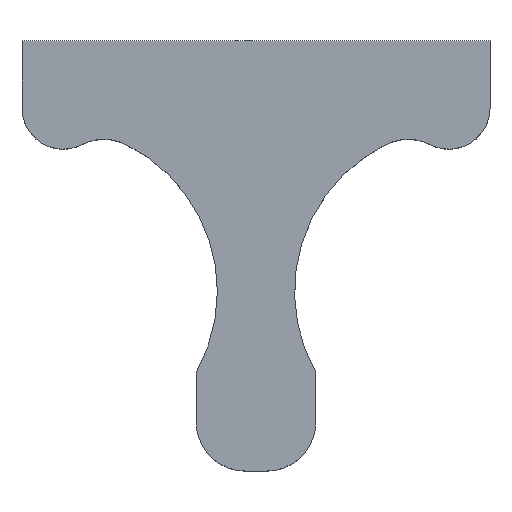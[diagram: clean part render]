
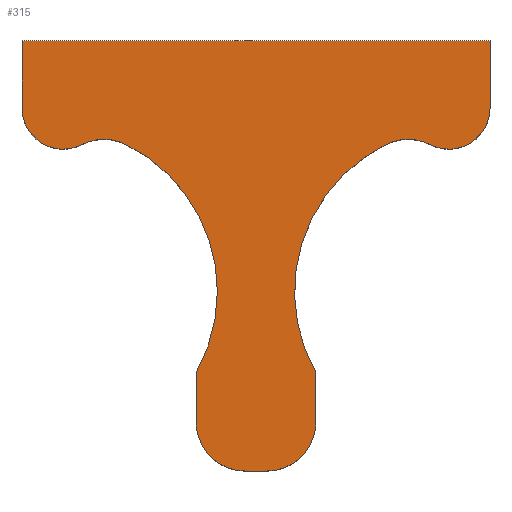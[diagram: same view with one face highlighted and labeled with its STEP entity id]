
A CAD part, top view. The second image highlights one B-rep face of the part: STEP entity #315.
In plain terms, the highlighted planar face has unit normal (0, 0, 1).
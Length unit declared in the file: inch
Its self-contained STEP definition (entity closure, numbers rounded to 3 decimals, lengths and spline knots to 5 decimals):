
#12 = EDGE_CURVE ( 'NONE', #204, #363, #301, .T. ) ;
#14 = DIRECTION ( 'NONE',  ( 0., 0., 1. ) ) ;
#17 = AXIS2_PLACEMENT_3D ( 'NONE', #470, #14, #563 ) ;
#20 = VERTEX_POINT ( 'NONE', #534 ) ;
#24 = EDGE_CURVE ( 'NONE', #46, #204, #52, .T. ) ;
#29 = CIRCLE ( 'NONE', #97, 0.03 ) ;
#37 = CARTESIAN_POINT ( 'NONE',  ( -0.1235, -0.15277, 0.026 ) ) ;
#38 = LINE ( 'NONE', #488, #371 ) ;
#46 = VERTEX_POINT ( 'NONE', #209 ) ;
#47 = DIRECTION ( 'NONE',  ( 0., 1., 0. ) ) ;
#49 = CARTESIAN_POINT ( 'NONE',  ( -0.1175, -0.041, 0.026 ) ) ;
#52 = CIRCLE ( 'NONE', #155, 0.03 ) ;
#54 = ORIENTED_EDGE ( 'NONE', *, *, #345, .T. ) ;
#62 = VERTEX_POINT ( 'NONE', #578 ) ;
#63 = EDGE_CURVE ( 'NONE', #366, #337, #443, .T. ) ;
#69 = VECTOR ( 'NONE', #482, 39.37008 ) ;
#70 = DIRECTION ( 'NONE',  ( 0., 0., 1. ) ) ;
#83 = DIRECTION ( 'NONE',  ( -1., 0., 0. ) ) ;
#84 = CARTESIAN_POINT ( 'NONE',  ( -0.1425, 0., 0.026 ) ) ;
#85 = VERTEX_POINT ( 'NONE', #167 ) ;
#91 = LINE ( 'NONE', #467, #316 ) ;
#93 = CIRCLE ( 'NONE', #390, 0.025 ) ;
#95 = CARTESIAN_POINT ( 'NONE',  ( 0.09252, -0.09, 0.026 ) ) ;
#97 = AXIS2_PLACEMENT_3D ( 'NONE', #405, #587, #306 ) ;
#99 = DIRECTION ( 'NONE',  ( 1., 0., 0. ) ) ;
#104 = VERTEX_POINT ( 'NONE', #84 ) ;
#114 = CARTESIAN_POINT ( 'NONE',  ( -0.0065, -0.262, 0.026 ) ) ;
#120 = CARTESIAN_POINT ( 'NONE',  ( -0.1175, -0.041, 0.026 ) ) ;
#126 = EDGE_CURVE ( 'NONE', #85, #62, #29, .T. ) ;
#130 = CARTESIAN_POINT ( 'NONE',  ( 0.0065, -0.262, 0.026 ) ) ;
#134 = EDGE_CURVE ( 'NONE', #62, #372, #589, .T. ) ;
#135 = VERTEX_POINT ( 'NONE', #496 ) ;
#136 = DIRECTION ( 'NONE',  ( 0., 0., 1. ) ) ;
#137 = DIRECTION ( 'NONE',  ( 0., 0., -1. ) ) ;
#138 = DIRECTION ( 'NONE',  ( 0., 0., 1. ) ) ;
#142 = CARTESIAN_POINT ( 'NONE',  ( 0.0365, -0.20208, 0.026 ) ) ;
#143 = AXIS2_PLACEMENT_3D ( 'NONE', #37, #446, #83 ) ;
#145 = AXIS2_PLACEMENT_3D ( 'NONE', #495, #299, #537 ) ;
#154 = DIRECTION ( 'NONE',  ( 0., -1., 0. ) ) ;
#155 = AXIS2_PLACEMENT_3D ( 'NONE', #309, #70, #402 ) ;
#165 = CARTESIAN_POINT ( 'NONE',  ( 0.1425, 0., 0.026 ) ) ;
#167 = CARTESIAN_POINT ( 'NONE',  ( -0.10615, -0.06327, 0.026 ) ) ;
#171 = VERTEX_POINT ( 'NONE', #413 ) ;
#201 = VECTOR ( 'NONE', #154, 39.37008 ) ;
#204 = VERTEX_POINT ( 'NONE', #403 ) ;
#208 = EDGE_CURVE ( 'NONE', #291, #135, #259, .T. ) ;
#209 = CARTESIAN_POINT ( 'NONE',  ( -0.0365, -0.232, 0.026 ) ) ;
#217 = CIRCLE ( 'NONE', #553, 0.025 ) ;
#225 = EDGE_CURVE ( 'NONE', #20, #366, #429, .T. ) ;
#232 = ORIENTED_EDGE ( 'NONE', *, *, #12, .T. ) ;
#240 = FACE_OUTER_BOUND ( 'NONE', #475, .T. ) ;
#244 = ORIENTED_EDGE ( 'NONE', *, *, #379, .T. ) ;
#259 = LINE ( 'NONE', #165, #562 ) ;
#261 = AXIS2_PLACEMENT_3D ( 'NONE', #49, #136, #281 ) ;
#268 = CARTESIAN_POINT ( 'NONE',  ( 0.1425, -0.041, 0.026 ) ) ;
#270 = PLANE ( 'NONE',  #261 ) ;
#272 = ORIENTED_EDGE ( 'NONE', *, *, #24, .T. ) ;
#275 = AXIS2_PLACEMENT_3D ( 'NONE', #95, #519, #99 ) ;
#276 = ORIENTED_EDGE ( 'NONE', *, *, #577, .T. ) ;
#281 = DIRECTION ( 'NONE',  ( 1., 0., 0. ) ) ;
#289 = LINE ( 'NONE', #440, #201 ) ;
#291 = VERTEX_POINT ( 'NONE', #268 ) ;
#293 = ORIENTED_EDGE ( 'NONE', *, *, #208, .T. ) ;
#299 = DIRECTION ( 'NONE',  ( 0., 0., -1. ) ) ;
#301 = LINE ( 'NONE', #114, #69 ) ;
#306 = DIRECTION ( 'NONE',  ( -1., 0., 0. ) ) ;
#309 = CARTESIAN_POINT ( 'NONE',  ( -0.0065, -0.232, 0.026 ) ) ;
#315 = ADVANCED_FACE ( 'NONE', ( #240 ), #270, .T. ) ;
#316 = VECTOR ( 'NONE', #421, 39.37008 ) ;
#317 = CARTESIAN_POINT ( 'NONE',  ( -0.0235, -0.15277, 0.026 ) ) ;
#318 = ORIENTED_EDGE ( 'NONE', *, *, #570, .T. ) ;
#323 = DIRECTION ( 'NONE',  ( -1., 0., 0. ) ) ;
#326 = CIRCLE ( 'NONE', #275, 0.03 ) ;
#328 = CARTESIAN_POINT ( 'NONE',  ( 0.1175, -0.041, 0.026 ) ) ;
#331 = ORIENTED_EDGE ( 'NONE', *, *, #490, .T. ) ;
#336 = AXIS2_PLACEMENT_3D ( 'NONE', #484, #137, #422 ) ;
#337 = VERTEX_POINT ( 'NONE', #511 ) ;
#345 = EDGE_CURVE ( 'NONE', #510, #46, #91, .T. ) ;
#347 = CIRCLE ( 'NONE', #17, 0.03 ) ;
#355 = DIRECTION ( 'NONE',  ( 0., 0., 1. ) ) ;
#363 = VERTEX_POINT ( 'NONE', #130 ) ;
#366 = VERTEX_POINT ( 'NONE', #142 ) ;
#369 = ORIENTED_EDGE ( 'NONE', *, *, #134, .T. ) ;
#371 = VECTOR ( 'NONE', #492, 39.37008 ) ;
#372 = VERTEX_POINT ( 'NONE', #317 ) ;
#379 = EDGE_CURVE ( 'NONE', #171, #291, #93, .T. ) ;
#380 = ORIENTED_EDGE ( 'NONE', *, *, #387, .T. ) ;
#387 = EDGE_CURVE ( 'NONE', #337, #171, #326, .T. ) ;
#390 = AXIS2_PLACEMENT_3D ( 'NONE', #328, #138, #323 ) ;
#402 = DIRECTION ( 'NONE',  ( 1., 0., 0. ) ) ;
#403 = CARTESIAN_POINT ( 'NONE',  ( -0.0065, -0.262, 0.026 ) ) ;
#405 = CARTESIAN_POINT ( 'NONE',  ( -0.09252, -0.09, 0.026 ) ) ;
#413 = CARTESIAN_POINT ( 'NONE',  ( 0.10615, -0.06327, 0.026 ) ) ;
#421 = DIRECTION ( 'NONE',  ( 0., -1., 0. ) ) ;
#422 = DIRECTION ( 'NONE',  ( -1., 0., 0. ) ) ;
#429 = LINE ( 'NONE', #515, #501 ) ;
#432 = EDGE_CURVE ( 'NONE', #104, #568, #289, .T. ) ;
#440 = CARTESIAN_POINT ( 'NONE',  ( -0.1425, 0., 0.026 ) ) ;
#443 = CIRCLE ( 'NONE', #145, 0.1 ) ;
#446 = DIRECTION ( 'NONE',  ( 0., 0., -1. ) ) ;
#447 = DIRECTION ( 'NONE',  ( 1., 0., 0. ) ) ;
#453 = CARTESIAN_POINT ( 'NONE',  ( -0.1425, -0.041, 0.026 ) ) ;
#467 = CARTESIAN_POINT ( 'NONE',  ( -0.0365, -0.20208, 0.026 ) ) ;
#470 = CARTESIAN_POINT ( 'NONE',  ( 0.0065, -0.232, 0.026 ) ) ;
#475 = EDGE_LOOP ( 'NONE', ( #514, #276, #499, #369, #331, #54, #272, #232, #504, #558, #486, #380, #244, #293, #318 ) ) ;
#482 = DIRECTION ( 'NONE',  ( 1., 0., 0. ) ) ;
#484 = CARTESIAN_POINT ( 'NONE',  ( -0.1235, -0.15277, 0.026 ) ) ;
#486 = ORIENTED_EDGE ( 'NONE', *, *, #63, .T. ) ;
#488 = CARTESIAN_POINT ( 'NONE',  ( -0.1425, 0., 0.026 ) ) ;
#490 = EDGE_CURVE ( 'NONE', #372, #510, #505, .T. ) ;
#492 = DIRECTION ( 'NONE',  ( -1., 0., 0. ) ) ;
#495 = CARTESIAN_POINT ( 'NONE',  ( 0.1235, -0.15277, 0.026 ) ) ;
#496 = CARTESIAN_POINT ( 'NONE',  ( 0.1425, 0., 0.026 ) ) ;
#499 = ORIENTED_EDGE ( 'NONE', *, *, #126, .T. ) ;
#501 = VECTOR ( 'NONE', #47, 39.37008 ) ;
#504 = ORIENTED_EDGE ( 'NONE', *, *, #533, .T. ) ;
#505 = CIRCLE ( 'NONE', #336, 0.1 ) ;
#510 = VERTEX_POINT ( 'NONE', #517 ) ;
#511 = CARTESIAN_POINT ( 'NONE',  ( 0.07924, -0.0631, 0.026 ) ) ;
#514 = ORIENTED_EDGE ( 'NONE', *, *, #432, .T. ) ;
#515 = CARTESIAN_POINT ( 'NONE',  ( 0.0365, -0.20208, 0.026 ) ) ;
#517 = CARTESIAN_POINT ( 'NONE',  ( -0.0365, -0.20208, 0.026 ) ) ;
#519 = DIRECTION ( 'NONE',  ( 0., 0., -1. ) ) ;
#533 = EDGE_CURVE ( 'NONE', #363, #20, #347, .T. ) ;
#534 = CARTESIAN_POINT ( 'NONE',  ( 0.0365, -0.232, 0.026 ) ) ;
#537 = DIRECTION ( 'NONE',  ( 1., 0., 0. ) ) ;
#540 = DIRECTION ( 'NONE',  ( 0., 1., 0. ) ) ;
#553 = AXIS2_PLACEMENT_3D ( 'NONE', #120, #355, #447 ) ;
#558 = ORIENTED_EDGE ( 'NONE', *, *, #225, .T. ) ;
#562 = VECTOR ( 'NONE', #540, 39.37008 ) ;
#563 = DIRECTION ( 'NONE',  ( -1., 0., 0. ) ) ;
#568 = VERTEX_POINT ( 'NONE', #453 ) ;
#570 = EDGE_CURVE ( 'NONE', #135, #104, #38, .T. ) ;
#577 = EDGE_CURVE ( 'NONE', #568, #85, #217, .T. ) ;
#578 = CARTESIAN_POINT ( 'NONE',  ( -0.07924, -0.0631, 0.026 ) ) ;
#587 = DIRECTION ( 'NONE',  ( 0., 0., -1. ) ) ;
#589 = CIRCLE ( 'NONE', #143, 0.1 ) ;
